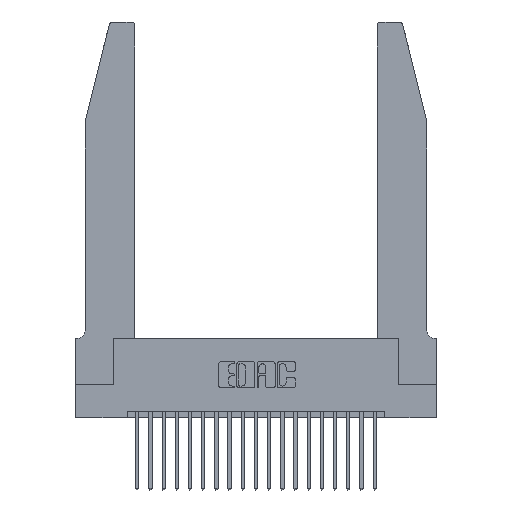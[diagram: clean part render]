
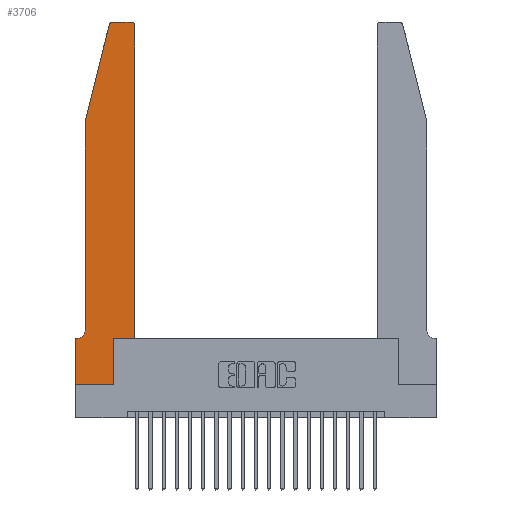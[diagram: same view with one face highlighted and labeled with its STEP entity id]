
A CAD part, top view. The second image highlights one B-rep face of the part: STEP entity #3706.
In plain terms, the highlighted planar face has unit normal (0, 0, 1).
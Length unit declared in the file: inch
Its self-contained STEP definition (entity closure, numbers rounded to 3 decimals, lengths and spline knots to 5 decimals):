
#133 = DIRECTION ( 'NONE',  ( 0., -1., 0. ) ) ;
#308 = LINE ( 'NONE', #21350, #3070 ) ;
#391 = DIRECTION ( 'NONE',  ( -1., 0., 0. ) ) ;
#857 = CARTESIAN_POINT ( 'NONE',  ( 0.0055, 0.42, 0.37 ) ) ;
#954 = CARTESIAN_POINT ( 'NONE',  ( 0., 0.35, 0.37 ) ) ;
#1353 = EDGE_CURVE ( 'NONE', #8483, #4190, #19835, .T. ) ;
#1376 = AXIS2_PLACEMENT_3D ( 'NONE', #1486, #13855, #17490 ) ;
#1486 = CARTESIAN_POINT ( 'NONE',  ( 0., 0.35, 0.37 ) ) ;
#1593 = DIRECTION ( 'NONE',  ( -1., 0., 0. ) ) ;
#2075 = LINE ( 'NONE', #10690, #6009 ) ;
#2089 = VERTEX_POINT ( 'NONE', #13648 ) ;
#2172 = VECTOR ( 'NONE', #3311, 39.37008 ) ;
#2248 = CARTESIAN_POINT ( 'NONE',  ( 0.4505, 0.35, 0.37 ) ) ;
#2588 = EDGE_CURVE ( 'NONE', #22003, #11193, #8020, .T. ) ;
#2727 = VECTOR ( 'NONE', #17404, 39.37008 ) ;
#2953 = FACE_OUTER_BOUND ( 'NONE', #13110, .T. ) ;
#3070 = VECTOR ( 'NONE', #11003, 39.37008 ) ;
#3112 = CARTESIAN_POINT ( 'NONE',  ( 0.284, 2.75, 0.37 ) ) ;
#3204 = DIRECTION ( 'NONE',  ( 1., 0., 0. ) ) ;
#3274 = CARTESIAN_POINT ( 'NONE',  ( 0.0055, 0.35, 0.37 ) ) ;
#3278 = EDGE_CURVE ( 'NONE', #21461, #11918, #13768, .T. ) ;
#3311 = DIRECTION ( 'NONE',  ( 1., 0., 0. ) ) ;
#3438 = CARTESIAN_POINT ( 'NONE',  ( 0.4505, 2.72, 0.37 ) ) ;
#3678 = AXIS2_PLACEMENT_3D ( 'NONE', #12545, #5522, #17867 ) ;
#3706 = ADVANCED_FACE ( 'NONE', ( #2953 ), #22436, .T. ) ;
#3734 = VERTEX_POINT ( 'NONE', #3112 ) ;
#4086 = DIRECTION ( 'NONE',  ( 0., 1., 0. ) ) ;
#4190 = VERTEX_POINT ( 'NONE', #3274 ) ;
#4372 = EDGE_CURVE ( 'NONE', #11006, #8483, #2075, .T. ) ;
#4989 = VERTEX_POINT ( 'NONE', #19705 ) ;
#5066 = ORIENTED_EDGE ( 'NONE', *, *, #1353, .T. ) ;
#5234 = VECTOR ( 'NONE', #9246, 39.37008 ) ;
#5459 = ORIENTED_EDGE ( 'NONE', *, *, #7249, .T. ) ;
#5522 = DIRECTION ( 'NONE',  ( 0., 0., 1. ) ) ;
#5823 = LINE ( 'NONE', #15952, #2172 ) ;
#6009 = VECTOR ( 'NONE', #133, 39.37008 ) ;
#6023 = ORIENTED_EDGE ( 'NONE', *, *, #19225, .T. ) ;
#6128 = CARTESIAN_POINT ( 'NONE',  ( 0.2865, 0.35, 0.37 ) ) ;
#6246 = VECTOR ( 'NONE', #16456, 39.37008 ) ;
#7016 = CARTESIAN_POINT ( 'NONE',  ( 0., 0., 0.37 ) ) ;
#7249 = EDGE_CURVE ( 'NONE', #2089, #14218, #19475, .T. ) ;
#7390 = CARTESIAN_POINT ( 'NONE',  ( 0.0755, 2., 0.37 ) ) ;
#8020 = LINE ( 'NONE', #20940, #2727 ) ;
#8483 = VERTEX_POINT ( 'NONE', #19944 ) ;
#8813 = CARTESIAN_POINT ( 'NONE',  ( 0.0755, 0.35, 0.37 ) ) ;
#9246 = DIRECTION ( 'NONE',  ( 0., 1., 0. ) ) ;
#9553 = EDGE_CURVE ( 'NONE', #11918, #4989, #12819, .T. ) ;
#9816 = LINE ( 'NONE', #7390, #6246 ) ;
#10072 = ORIENTED_EDGE ( 'NONE', *, *, #14713, .T. ) ;
#10097 = AXIS2_PLACEMENT_3D ( 'NONE', #857, #21936, #391 ) ;
#10168 = VECTOR ( 'NONE', #4086, 39.37008 ) ;
#10248 = CARTESIAN_POINT ( 'NONE',  ( 0.284, 2.72, 0.37 ) ) ;
#10690 = CARTESIAN_POINT ( 'NONE',  ( 0.0755, 2., 0.37 ) ) ;
#11003 = DIRECTION ( 'NONE',  ( 1., 0., 0. ) ) ;
#11006 = VERTEX_POINT ( 'NONE', #22161 ) ;
#11193 = VERTEX_POINT ( 'NONE', #7016 ) ;
#11211 = ORIENTED_EDGE ( 'NONE', *, *, #9553, .T. ) ;
#11294 = VECTOR ( 'NONE', #1593, 39.37008 ) ;
#11368 = VERTEX_POINT ( 'NONE', #15159 ) ;
#11471 = VECTOR ( 'NONE', #21529, 39.37008 ) ;
#11839 = EDGE_CURVE ( 'NONE', #3734, #11368, #17368, .T. ) ;
#11918 = VERTEX_POINT ( 'NONE', #3438 ) ;
#12545 = CARTESIAN_POINT ( 'NONE',  ( 0.4205, 2.72, 0.37 ) ) ;
#12819 = CIRCLE ( 'NONE', #3678, 0.03 ) ;
#12966 = EDGE_CURVE ( 'NONE', #4989, #3734, #14870, .T. ) ;
#13110 = EDGE_LOOP ( 'NONE', ( #21544, #20414, #6023, #15280, #5066, #21728, #21929, #19899, #5459, #10072, #20434, #11211 ) ) ;
#13648 = CARTESIAN_POINT ( 'NONE',  ( 0.2865, 0., 0.37 ) ) ;
#13768 = LINE ( 'NONE', #2248, #5234 ) ;
#13794 = DIRECTION ( 'NONE',  ( 0., 0., 1. ) ) ;
#13815 = CARTESIAN_POINT ( 'NONE',  ( 0.2605, 2.75, 0.37 ) ) ;
#13855 = DIRECTION ( 'NONE',  ( 0., 0., 1. ) ) ;
#14218 = VERTEX_POINT ( 'NONE', #22642 ) ;
#14478 = LINE ( 'NONE', #8813, #11471 ) ;
#14713 = EDGE_CURVE ( 'NONE', #14218, #21461, #308, .T. ) ;
#14752 = AXIS2_PLACEMENT_3D ( 'NONE', #10248, #13794, #3204 ) ;
#14870 = LINE ( 'NONE', #13815, #11294 ) ;
#15159 = CARTESIAN_POINT ( 'NONE',  ( 0.25487, 2.72718, 0.37 ) ) ;
#15280 = ORIENTED_EDGE ( 'NONE', *, *, #4372, .T. ) ;
#15952 = CARTESIAN_POINT ( 'NONE',  ( 0., 0., 0.37 ) ) ;
#16456 = DIRECTION ( 'NONE',  ( -0.239, -0.971, 0. ) ) ;
#17368 = CIRCLE ( 'NONE', #14752, 0.03 ) ;
#17404 = DIRECTION ( 'NONE',  ( 0., -1., 0. ) ) ;
#17490 = DIRECTION ( 'NONE',  ( 1., 0., 0. ) ) ;
#17867 = DIRECTION ( 'NONE',  ( 1., 0., 0. ) ) ;
#18441 = CARTESIAN_POINT ( 'NONE',  ( 0.4505, 0.35, 0.37 ) ) ;
#18513 = EDGE_CURVE ( 'NONE', #4190, #22003, #14478, .T. ) ;
#19225 = EDGE_CURVE ( 'NONE', #11368, #11006, #9816, .T. ) ;
#19475 = LINE ( 'NONE', #6128, #10168 ) ;
#19705 = CARTESIAN_POINT ( 'NONE',  ( 0.4205, 2.75, 0.37 ) ) ;
#19835 = CIRCLE ( 'NONE', #10097, 0.07 ) ;
#19899 = ORIENTED_EDGE ( 'NONE', *, *, #21167, .T. ) ;
#19944 = CARTESIAN_POINT ( 'NONE',  ( 0.0755, 0.42, 0.37 ) ) ;
#20414 = ORIENTED_EDGE ( 'NONE', *, *, #11839, .T. ) ;
#20434 = ORIENTED_EDGE ( 'NONE', *, *, #3278, .T. ) ;
#20940 = CARTESIAN_POINT ( 'NONE',  ( 0., 0., 0.37 ) ) ;
#21167 = EDGE_CURVE ( 'NONE', #11193, #2089, #5823, .T. ) ;
#21350 = CARTESIAN_POINT ( 'NONE',  ( 0.4505, 0.35, 0.37 ) ) ;
#21461 = VERTEX_POINT ( 'NONE', #18441 ) ;
#21529 = DIRECTION ( 'NONE',  ( -1., 0., 0. ) ) ;
#21544 = ORIENTED_EDGE ( 'NONE', *, *, #12966, .T. ) ;
#21728 = ORIENTED_EDGE ( 'NONE', *, *, #18513, .T. ) ;
#21929 = ORIENTED_EDGE ( 'NONE', *, *, #2588, .T. ) ;
#21936 = DIRECTION ( 'NONE',  ( 0., 0., -1. ) ) ;
#22003 = VERTEX_POINT ( 'NONE', #954 ) ;
#22161 = CARTESIAN_POINT ( 'NONE',  ( 0.0755, 2., 0.37 ) ) ;
#22436 = PLANE ( 'NONE',  #1376 ) ;
#22642 = CARTESIAN_POINT ( 'NONE',  ( 0.2865, 0.35, 0.37 ) ) ;
